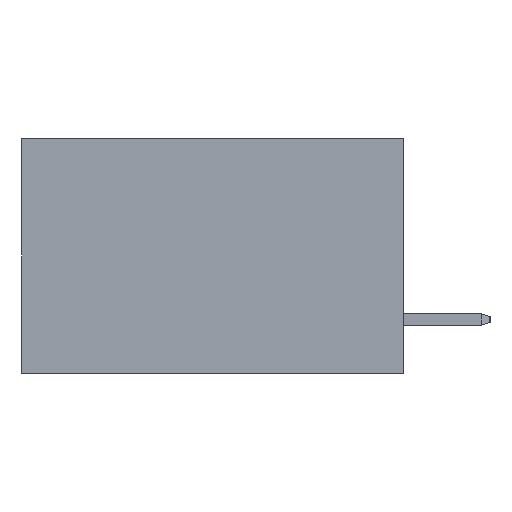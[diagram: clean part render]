
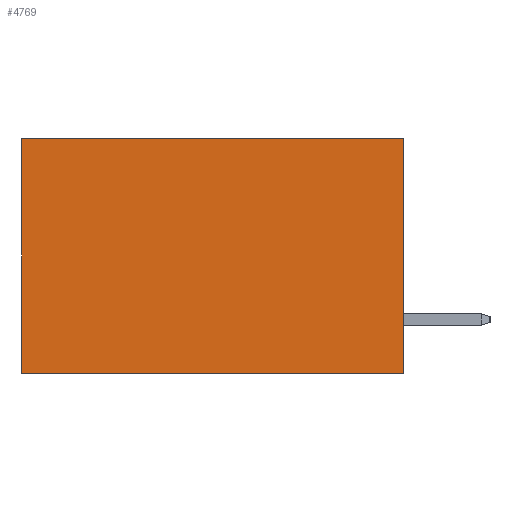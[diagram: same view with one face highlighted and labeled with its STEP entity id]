
A CAD part, left-side view. The second image highlights one B-rep face of the part: STEP entity #4769.
In plain terms, the highlighted planar face has unit normal (-1, 0, 0).
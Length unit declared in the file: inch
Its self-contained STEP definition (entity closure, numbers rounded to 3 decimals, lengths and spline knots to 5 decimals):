
#1285 = CARTESIAN_POINT ( 'NONE',  ( 0.2875, 0., 0. ) ) ;
#1435 = DIRECTION ( 'NONE',  ( 1., 0., 0. ) ) ;
#1651 = DIRECTION ( 'NONE',  ( 0., 0., -1. ) ) ;
#1815 = DIRECTION ( 'NONE',  ( 0., 1., 0. ) ) ;
#1830 = VERTEX_POINT ( 'NONE', #14426 ) ;
#1844 = ORIENTED_EDGE ( 'NONE', *, *, #4237, .T. ) ;
#3826 = LINE ( 'NONE', #8394, #14491 ) ;
#4132 = VERTEX_POINT ( 'NONE', #5707 ) ;
#4237 = EDGE_CURVE ( 'NONE', #9439, #1830, #3826, .T. ) ;
#4272 = CARTESIAN_POINT ( 'NONE',  ( 0.2875, 0., 0. ) ) ;
#4769 = ADVANCED_FACE ( 'NONE', ( #6283 ), #11644, .F. ) ;
#4772 = EDGE_CURVE ( 'NONE', #4132, #5908, #6142, .T. ) ;
#5097 = ORIENTED_EDGE ( 'NONE', *, *, #11985, .F. ) ;
#5707 = CARTESIAN_POINT ( 'NONE',  ( 0.2875, 0., -0.37 ) ) ;
#5908 = VERTEX_POINT ( 'NONE', #6538 ) ;
#6142 = LINE ( 'NONE', #9412, #11273 ) ;
#6283 = FACE_OUTER_BOUND ( 'NONE', #8010, .T. ) ;
#6392 = EDGE_CURVE ( 'NONE', #1830, #5908, #14707, .T. ) ;
#6538 = CARTESIAN_POINT ( 'NONE',  ( 0.2875, 0.6, -0.37 ) ) ;
#6599 = CARTESIAN_POINT ( 'NONE',  ( 0.2875, 0.6, 0. ) ) ;
#6816 = LINE ( 'NONE', #4272, #9032 ) ;
#7702 = ORIENTED_EDGE ( 'NONE', *, *, #4772, .F. ) ;
#8010 = EDGE_LOOP ( 'NONE', ( #12311, #7702, #5097, #1844 ) ) ;
#8394 = CARTESIAN_POINT ( 'NONE',  ( 0.2875, 0., 0. ) ) ;
#9032 = VECTOR ( 'NONE', #11360, 39.37008 ) ;
#9412 = CARTESIAN_POINT ( 'NONE',  ( 0.2875, 0., -0.37 ) ) ;
#9439 = VERTEX_POINT ( 'NONE', #1285 ) ;
#9631 = VECTOR ( 'NONE', #11137, 39.37008 ) ;
#10272 = AXIS2_PLACEMENT_3D ( 'NONE', #12908, #1435, #1651 ) ;
#10819 = DIRECTION ( 'NONE',  ( 0., 1., 0. ) ) ;
#11137 = DIRECTION ( 'NONE',  ( 0., 0., -1. ) ) ;
#11273 = VECTOR ( 'NONE', #10819, 39.37008 ) ;
#11360 = DIRECTION ( 'NONE',  ( 0., 0., -1. ) ) ;
#11644 = PLANE ( 'NONE',  #10272 ) ;
#11985 = EDGE_CURVE ( 'NONE', #9439, #4132, #6816, .T. ) ;
#12311 = ORIENTED_EDGE ( 'NONE', *, *, #6392, .T. ) ;
#12908 = CARTESIAN_POINT ( 'NONE',  ( 0.2875, 0., 0. ) ) ;
#14426 = CARTESIAN_POINT ( 'NONE',  ( 0.2875, 0.6, 0. ) ) ;
#14491 = VECTOR ( 'NONE', #1815, 39.37008 ) ;
#14707 = LINE ( 'NONE', #6599, #9631 ) ;
